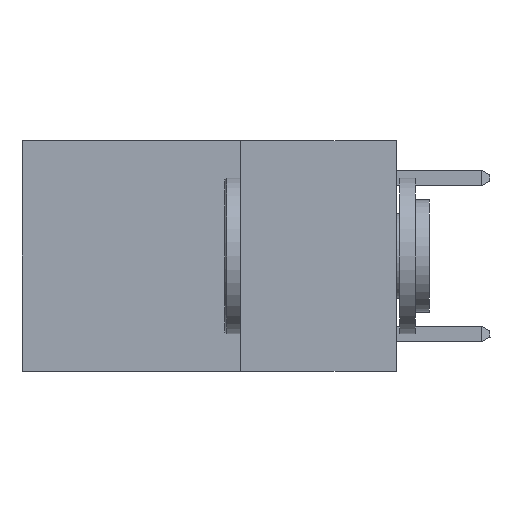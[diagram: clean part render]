
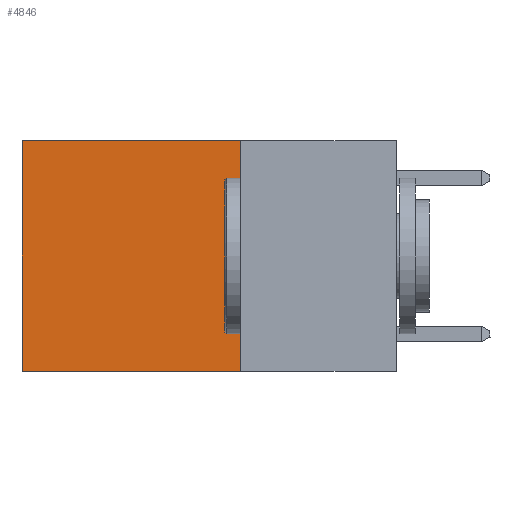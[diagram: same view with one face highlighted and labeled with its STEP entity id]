
A CAD part, left-side view. The second image highlights one B-rep face of the part: STEP entity #4846.
In plain terms, the highlighted planar face has unit normal (-1, 0, 0).
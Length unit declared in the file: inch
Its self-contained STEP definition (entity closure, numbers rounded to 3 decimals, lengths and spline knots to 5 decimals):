
#101 = DIRECTION ( 'NONE',  ( 0., 1., 0. ) ) ;
#113 = EDGE_CURVE ( 'NONE', #7784, #1428, #10850, .T. ) ;
#868 = ORIENTED_EDGE ( 'NONE', *, *, #10601, .F. ) ;
#904 = PLANE ( 'NONE',  #7976 ) ;
#1009 = CARTESIAN_POINT ( 'NONE',  ( 0.2625, 0.25, 0. ) ) ;
#1048 = VECTOR ( 'NONE', #8704, 39.37008 ) ;
#1049 = VECTOR ( 'NONE', #10145, 39.37008 ) ;
#1428 = VERTEX_POINT ( 'NONE', #8594 ) ;
#1454 = VECTOR ( 'NONE', #101, 39.37008 ) ;
#1659 = ORIENTED_EDGE ( 'NONE', *, *, #113, .T. ) ;
#1881 = CARTESIAN_POINT ( 'NONE',  ( 0.2625, 0.25, 0. ) ) ;
#2135 = ORIENTED_EDGE ( 'NONE', *, *, #8479, .F. ) ;
#2257 = VERTEX_POINT ( 'NONE', #6491 ) ;
#2779 = LINE ( 'NONE', #1881, #1049 ) ;
#2803 = LINE ( 'NONE', #4461, #3479 ) ;
#2829 = FACE_OUTER_BOUND ( 'NONE', #5184, .T. ) ;
#2956 = CARTESIAN_POINT ( 'NONE',  ( 0.2625, 0.25, 0. ) ) ;
#3479 = VECTOR ( 'NONE', #8039, 39.37008 ) ;
#4078 = VERTEX_POINT ( 'NONE', #8286 ) ;
#4461 = CARTESIAN_POINT ( 'NONE',  ( 0.2625, 0.25, -0.37 ) ) ;
#4846 = ADVANCED_FACE ( 'NONE', ( #2829 ), #904, .F. ) ;
#5107 = LINE ( 'NONE', #10364, #1048 ) ;
#5184 = EDGE_LOOP ( 'NONE', ( #8795, #868, #2135, #1659 ) ) ;
#6491 = CARTESIAN_POINT ( 'NONE',  ( 0.2625, 0.25, -0.37 ) ) ;
#6995 = CARTESIAN_POINT ( 'NONE',  ( 0.2625, 0.25, 0. ) ) ;
#7784 = VERTEX_POINT ( 'NONE', #6995 ) ;
#7976 = AXIS2_PLACEMENT_3D ( 'NONE', #1009, #8304, #9232 ) ;
#8039 = DIRECTION ( 'NONE',  ( 0., 1., 0. ) ) ;
#8286 = CARTESIAN_POINT ( 'NONE',  ( 0.2625, 0.6, -0.37 ) ) ;
#8304 = DIRECTION ( 'NONE',  ( 1., 0., 0. ) ) ;
#8479 = EDGE_CURVE ( 'NONE', #7784, #2257, #2779, .T. ) ;
#8594 = CARTESIAN_POINT ( 'NONE',  ( 0.2625, 0.6, 0. ) ) ;
#8704 = DIRECTION ( 'NONE',  ( 0., 0., -1. ) ) ;
#8795 = ORIENTED_EDGE ( 'NONE', *, *, #10117, .T. ) ;
#9232 = DIRECTION ( 'NONE',  ( 0., 0., -1. ) ) ;
#10117 = EDGE_CURVE ( 'NONE', #1428, #4078, #5107, .T. ) ;
#10145 = DIRECTION ( 'NONE',  ( 0., 0., -1. ) ) ;
#10364 = CARTESIAN_POINT ( 'NONE',  ( 0.2625, 0.6, 0. ) ) ;
#10601 = EDGE_CURVE ( 'NONE', #2257, #4078, #2803, .T. ) ;
#10850 = LINE ( 'NONE', #2956, #1454 ) ;
